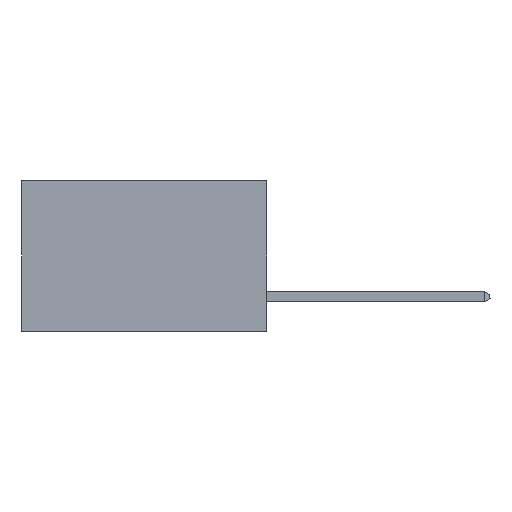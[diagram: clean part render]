
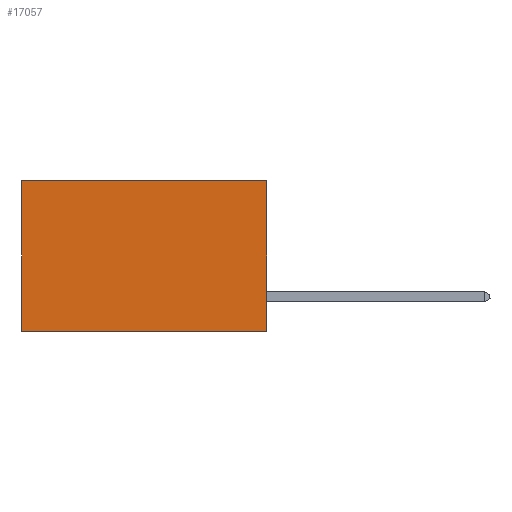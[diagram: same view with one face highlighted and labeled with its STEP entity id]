
A CAD part, left-side view. The second image highlights one B-rep face of the part: STEP entity #17057.
In plain terms, the highlighted planar face has unit normal (-1, 0, 0).
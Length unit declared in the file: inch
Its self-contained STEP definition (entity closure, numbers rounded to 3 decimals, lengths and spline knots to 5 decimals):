
#357 = CARTESIAN_POINT ( 'NONE',  ( 0.2875, 0., 0. ) ) ;
#881 = PLANE ( 'NONE',  #14619 ) ;
#965 = DIRECTION ( 'NONE',  ( 0., 0., -1. ) ) ;
#1075 = CARTESIAN_POINT ( 'NONE',  ( 0.2875, 0.6, -0.37 ) ) ;
#2692 = VERTEX_POINT ( 'NONE', #1075 ) ;
#2821 = CARTESIAN_POINT ( 'NONE',  ( 0.2875, 0., 0. ) ) ;
#3191 = DIRECTION ( 'NONE',  ( 0., 0., -1. ) ) ;
#3219 = LINE ( 'NONE', #25823, #24297 ) ;
#3840 = CARTESIAN_POINT ( 'NONE',  ( 0.2875, 0.6, 0. ) ) ;
#4110 = EDGE_CURVE ( 'NONE', #19246, #15590, #14362, .T. ) ;
#4642 = EDGE_LOOP ( 'NONE', ( #19588, #22047, #6442, #14895 ) ) ;
#5551 = CARTESIAN_POINT ( 'NONE',  ( 0.2875, 0.6, 0. ) ) ;
#6137 = LINE ( 'NONE', #24654, #6465 ) ;
#6442 = ORIENTED_EDGE ( 'NONE', *, *, #4110, .F. ) ;
#6465 = VECTOR ( 'NONE', #8426, 39.37008 ) ;
#8426 = DIRECTION ( 'NONE',  ( 0., 1., 0. ) ) ;
#8975 = VECTOR ( 'NONE', #3191, 39.37008 ) ;
#9829 = VECTOR ( 'NONE', #15978, 39.37008 ) ;
#10620 = FACE_OUTER_BOUND ( 'NONE', #4642, .T. ) ;
#14155 = EDGE_CURVE ( 'NONE', #16669, #2692, #18761, .T. ) ;
#14362 = LINE ( 'NONE', #21950, #8975 ) ;
#14619 = AXIS2_PLACEMENT_3D ( 'NONE', #2821, #23097, #965 ) ;
#14895 = ORIENTED_EDGE ( 'NONE', *, *, #18363, .T. ) ;
#15590 = VERTEX_POINT ( 'NONE', #19777 ) ;
#15978 = DIRECTION ( 'NONE',  ( 0., 0., -1. ) ) ;
#16669 = VERTEX_POINT ( 'NONE', #3840 ) ;
#17057 = ADVANCED_FACE ( 'NONE', ( #10620 ), #881, .F. ) ;
#18363 = EDGE_CURVE ( 'NONE', #19246, #16669, #6137, .T. ) ;
#18761 = LINE ( 'NONE', #5551, #9829 ) ;
#19182 = EDGE_CURVE ( 'NONE', #15590, #2692, #3219, .T. ) ;
#19246 = VERTEX_POINT ( 'NONE', #357 ) ;
#19588 = ORIENTED_EDGE ( 'NONE', *, *, #14155, .T. ) ;
#19757 = DIRECTION ( 'NONE',  ( 0., 1., 0. ) ) ;
#19777 = CARTESIAN_POINT ( 'NONE',  ( 0.2875, 0., -0.37 ) ) ;
#21950 = CARTESIAN_POINT ( 'NONE',  ( 0.2875, 0., 0. ) ) ;
#22047 = ORIENTED_EDGE ( 'NONE', *, *, #19182, .F. ) ;
#23097 = DIRECTION ( 'NONE',  ( 1., 0., 0. ) ) ;
#24297 = VECTOR ( 'NONE', #19757, 39.37008 ) ;
#24654 = CARTESIAN_POINT ( 'NONE',  ( 0.2875, 0., 0. ) ) ;
#25823 = CARTESIAN_POINT ( 'NONE',  ( 0.2875, 0., -0.37 ) ) ;
